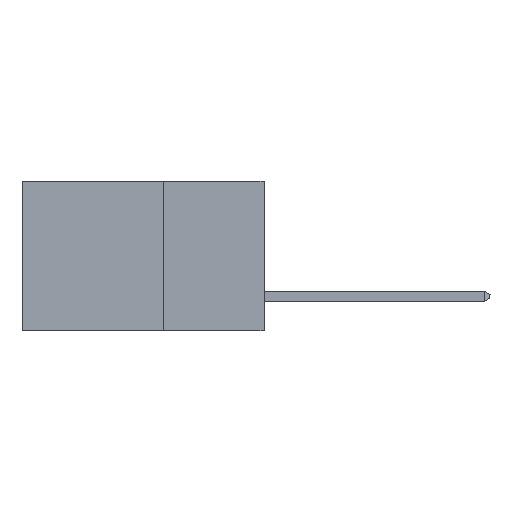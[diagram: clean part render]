
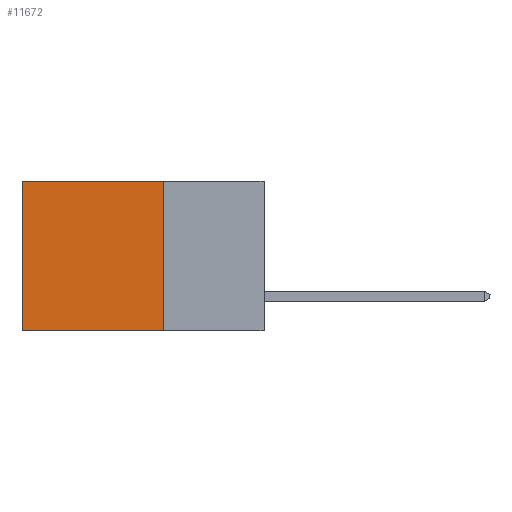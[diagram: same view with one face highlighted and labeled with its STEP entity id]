
A CAD part, left-side view. The second image highlights one B-rep face of the part: STEP entity #11672.
In plain terms, the highlighted planar face has unit normal (-1, 0, 0).
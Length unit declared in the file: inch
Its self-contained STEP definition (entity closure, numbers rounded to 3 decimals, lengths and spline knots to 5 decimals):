
#181 = DIRECTION ( 'NONE',  ( 0., 0., -1. ) ) ;
#1049 = LINE ( 'NONE', #23252, #17194 ) ;
#1450 = CARTESIAN_POINT ( 'NONE',  ( 0.298, 0.6, -0.37 ) ) ;
#2238 = VECTOR ( 'NONE', #9647, 39.37008 ) ;
#2378 = EDGE_CURVE ( 'NONE', #20877, #14103, #21062, .T. ) ;
#4476 = CARTESIAN_POINT ( 'NONE',  ( 0.298, 0.25, -0.37 ) ) ;
#5225 = VECTOR ( 'NONE', #18539, 39.37008 ) ;
#7145 = EDGE_LOOP ( 'NONE', ( #15238, #22148, #19319, #13415 ) ) ;
#9647 = DIRECTION ( 'NONE',  ( 0., 1., 0. ) ) ;
#9911 = VERTEX_POINT ( 'NONE', #17422 ) ;
#9994 = VERTEX_POINT ( 'NONE', #1450 ) ;
#10040 = EDGE_CURVE ( 'NONE', #14103, #9994, #17018, .T. ) ;
#10961 = CARTESIAN_POINT ( 'NONE',  ( 0.298, 0.25, -0.37 ) ) ;
#11672 = ADVANCED_FACE ( 'NONE', ( #22975 ), #14423, .F. ) ;
#12783 = CARTESIAN_POINT ( 'NONE',  ( 0.298, 0.25, 0. ) ) ;
#13415 = ORIENTED_EDGE ( 'NONE', *, *, #21685, .T. ) ;
#14103 = VERTEX_POINT ( 'NONE', #4476 ) ;
#14423 = PLANE ( 'NONE',  #15006 ) ;
#14763 = CARTESIAN_POINT ( 'NONE',  ( 0.298, 0.25, 0. ) ) ;
#15006 = AXIS2_PLACEMENT_3D ( 'NONE', #14763, #16657, #20357 ) ;
#15238 = ORIENTED_EDGE ( 'NONE', *, *, #20811, .T. ) ;
#16178 = VECTOR ( 'NONE', #181, 39.37008 ) ;
#16657 = DIRECTION ( 'NONE',  ( 1., 0., 0. ) ) ;
#16671 = LINE ( 'NONE', #20672, #2238 ) ;
#17018 = LINE ( 'NONE', #10961, #5225 ) ;
#17194 = VECTOR ( 'NONE', #17796, 39.37008 ) ;
#17422 = CARTESIAN_POINT ( 'NONE',  ( 0.298, 0.6, 0. ) ) ;
#17796 = DIRECTION ( 'NONE',  ( 0., 0., -1. ) ) ;
#18036 = CARTESIAN_POINT ( 'NONE',  ( 0.298, 0.25, 0. ) ) ;
#18539 = DIRECTION ( 'NONE',  ( 0., 1., 0. ) ) ;
#19319 = ORIENTED_EDGE ( 'NONE', *, *, #2378, .F. ) ;
#20357 = DIRECTION ( 'NONE',  ( 0., 0., -1. ) ) ;
#20672 = CARTESIAN_POINT ( 'NONE',  ( 0.298, 0.25, 0. ) ) ;
#20811 = EDGE_CURVE ( 'NONE', #9911, #9994, #1049, .T. ) ;
#20877 = VERTEX_POINT ( 'NONE', #18036 ) ;
#21062 = LINE ( 'NONE', #12783, #16178 ) ;
#21685 = EDGE_CURVE ( 'NONE', #20877, #9911, #16671, .T. ) ;
#22148 = ORIENTED_EDGE ( 'NONE', *, *, #10040, .F. ) ;
#22975 = FACE_OUTER_BOUND ( 'NONE', #7145, .T. ) ;
#23252 = CARTESIAN_POINT ( 'NONE',  ( 0.298, 0.6, 0. ) ) ;
